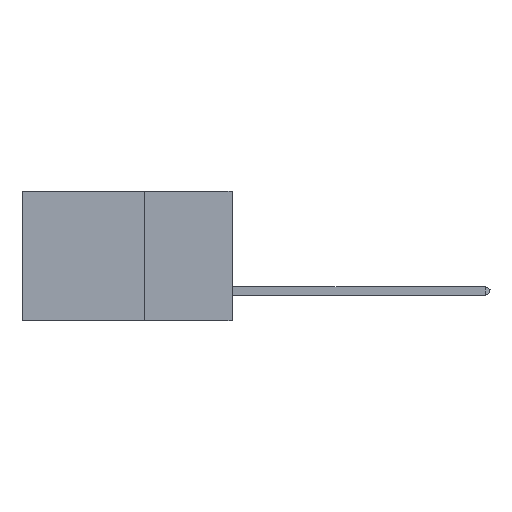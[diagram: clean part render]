
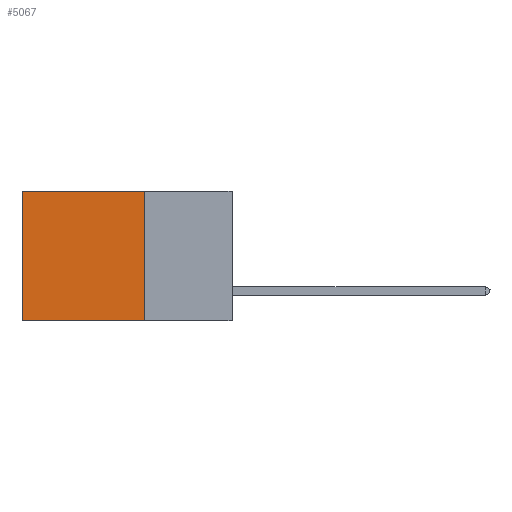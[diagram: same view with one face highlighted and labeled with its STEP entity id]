
A CAD part, left-side view. The second image highlights one B-rep face of the part: STEP entity #5067.
In plain terms, the highlighted planar face has unit normal (-1, 0, 0).
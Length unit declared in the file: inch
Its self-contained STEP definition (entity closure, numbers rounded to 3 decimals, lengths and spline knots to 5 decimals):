
#1588 = CARTESIAN_POINT ( 'NONE',  ( 0.2875, 0.25, 0. ) ) ;
#3718 = CARTESIAN_POINT ( 'NONE',  ( 0.2875, 0.25, 0. ) ) ;
#5067 = ADVANCED_FACE ( 'NONE', ( #28622 ), #27133, .F. ) ;
#7646 = CARTESIAN_POINT ( 'NONE',  ( 0.2875, 0.25, -0.37 ) ) ;
#8318 = VERTEX_POINT ( 'NONE', #7646 ) ;
#8784 = LINE ( 'NONE', #43938, #19803 ) ;
#10476 = VECTOR ( 'NONE', #48134, 39.37008 ) ;
#12285 = EDGE_CURVE ( 'NONE', #8318, #49360, #8784, .T. ) ;
#14183 = EDGE_CURVE ( 'NONE', #45912, #8318, #47492, .T. ) ;
#14195 = CARTESIAN_POINT ( 'NONE',  ( 0.2875, 0.25, 0. ) ) ;
#14986 = EDGE_LOOP ( 'NONE', ( #21716, #47549, #26356, #19868 ) ) ;
#14997 = LINE ( 'NONE', #22933, #24090 ) ;
#15416 = VERTEX_POINT ( 'NONE', #24111 ) ;
#19803 = VECTOR ( 'NONE', #32492, 39.37008 ) ;
#19819 = VECTOR ( 'NONE', #29765, 39.37008 ) ;
#19868 = ORIENTED_EDGE ( 'NONE', *, *, #46184, .T. ) ;
#21716 = ORIENTED_EDGE ( 'NONE', *, *, #38937, .T. ) ;
#22933 = CARTESIAN_POINT ( 'NONE',  ( 0.2875, 0.6, 0. ) ) ;
#23160 = AXIS2_PLACEMENT_3D ( 'NONE', #3718, #34974, #47238 ) ;
#24090 = VECTOR ( 'NONE', #50157, 39.37008 ) ;
#24111 = CARTESIAN_POINT ( 'NONE',  ( 0.2875, 0.6, 0. ) ) ;
#26356 = ORIENTED_EDGE ( 'NONE', *, *, #14183, .F. ) ;
#27133 = PLANE ( 'NONE',  #23160 ) ;
#28622 = FACE_OUTER_BOUND ( 'NONE', #14986, .T. ) ;
#29765 = DIRECTION ( 'NONE',  ( 0., 1., 0. ) ) ;
#31235 = CARTESIAN_POINT ( 'NONE',  ( 0.2875, 0.6, -0.37 ) ) ;
#32417 = CARTESIAN_POINT ( 'NONE',  ( 0.2875, 0.25, 0. ) ) ;
#32492 = DIRECTION ( 'NONE',  ( 0., 1., 0. ) ) ;
#34974 = DIRECTION ( 'NONE',  ( 1., 0., 0. ) ) ;
#38937 = EDGE_CURVE ( 'NONE', #15416, #49360, #14997, .T. ) ;
#43938 = CARTESIAN_POINT ( 'NONE',  ( 0.2875, 0.25, -0.37 ) ) ;
#45912 = VERTEX_POINT ( 'NONE', #32417 ) ;
#46184 = EDGE_CURVE ( 'NONE', #45912, #15416, #48360, .T. ) ;
#47238 = DIRECTION ( 'NONE',  ( 0., 0., -1. ) ) ;
#47492 = LINE ( 'NONE', #1588, #10476 ) ;
#47549 = ORIENTED_EDGE ( 'NONE', *, *, #12285, .F. ) ;
#48134 = DIRECTION ( 'NONE',  ( 0., 0., -1. ) ) ;
#48360 = LINE ( 'NONE', #14195, #19819 ) ;
#49360 = VERTEX_POINT ( 'NONE', #31235 ) ;
#50157 = DIRECTION ( 'NONE',  ( 0., 0., -1. ) ) ;
